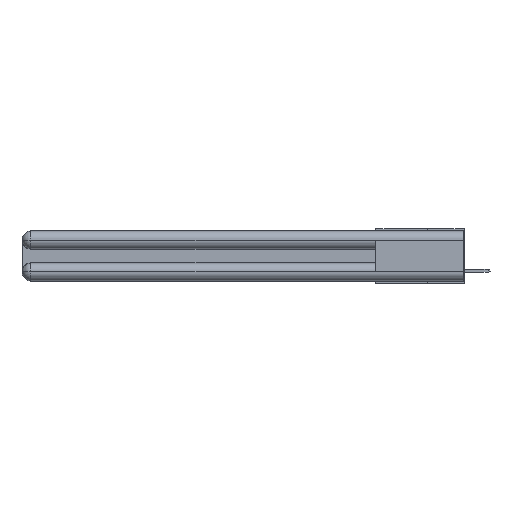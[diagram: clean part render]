
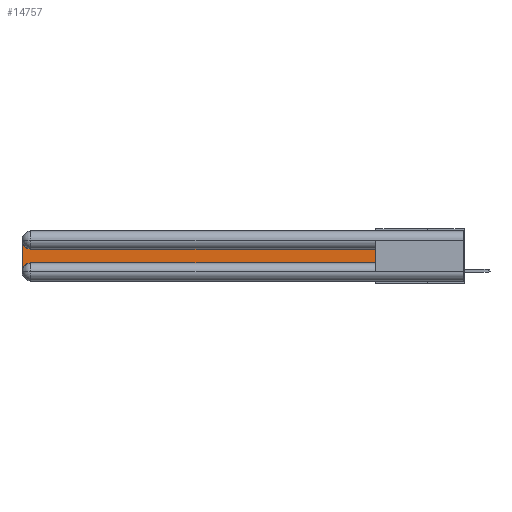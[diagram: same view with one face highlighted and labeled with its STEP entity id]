
A CAD part, left-side view. The second image highlights one B-rep face of the part: STEP entity #14757.
In plain terms, the highlighted planar face has unit normal (-1, 0, 0).
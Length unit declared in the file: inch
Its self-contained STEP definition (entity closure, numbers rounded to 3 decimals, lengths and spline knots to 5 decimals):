
#2024 = EDGE_LOOP ( 'NONE', ( #2301, #30990, #30283, #21975, #24722, #20316 ) ) ;
#2221 = CARTESIAN_POINT ( 'NONE',  ( 0.075, 3., -0.0625 ) ) ;
#2287 = AXIS2_PLACEMENT_3D ( 'NONE', #23627, #3652, #10839 ) ;
#2301 = ORIENTED_EDGE ( 'NONE', *, *, #5754, .T. ) ;
#2393 = VECTOR ( 'NONE', #24924, 39.37008 ) ;
#2893 = LINE ( 'NONE', #19226, #31942 ) ;
#3136 = DIRECTION ( 'NONE',  ( 0., 0., -1. ) ) ;
#3536 = EDGE_CURVE ( 'NONE', #25233, #27557, #24009, .T. ) ;
#3552 = DIRECTION ( 'NONE',  ( 0., 0., -1. ) ) ;
#3652 = DIRECTION ( 'NONE',  ( 1., 0., 0. ) ) ;
#4412 = EDGE_CURVE ( 'NONE', #13787, #19863, #2893, .T. ) ;
#5197 = EDGE_CURVE ( 'NONE', #27557, #18472, #24568, .T. ) ;
#5565 = AXIS2_PLACEMENT_3D ( 'NONE', #30758, #15905, #3552 ) ;
#5754 = EDGE_CURVE ( 'NONE', #18472, #8360, #21845, .T. ) ;
#6960 = EDGE_CURVE ( 'NONE', #8360, #13787, #17496, .T. ) ;
#7767 = CARTESIAN_POINT ( 'NONE',  ( 0.075, 0.6, -0.2175 ) ) ;
#8360 = VERTEX_POINT ( 'NONE', #31097 ) ;
#10649 = DIRECTION ( 'NONE',  ( 0., 0., 1. ) ) ;
#10839 = DIRECTION ( 'NONE',  ( 0., 0., -1. ) ) ;
#13787 = VERTEX_POINT ( 'NONE', #2221 ) ;
#13825 = AXIS2_PLACEMENT_3D ( 'NONE', #22681, #27758, #3136 ) ;
#14757 = ADVANCED_FACE ( 'NONE', ( #28942 ), #28274, .F. ) ;
#15905 = DIRECTION ( 'NONE',  ( 1., 0., 0. ) ) ;
#16246 = CIRCLE ( 'NONE', #5565, 0.06 ) ;
#17496 = CIRCLE ( 'NONE', #13825, 0.06 ) ;
#18472 = VERTEX_POINT ( 'NONE', #29125 ) ;
#19007 = DIRECTION ( 'NONE',  ( 0., 0., -1. ) ) ;
#19226 = CARTESIAN_POINT ( 'NONE',  ( 0.075, 3., -0.2175 ) ) ;
#19616 = CARTESIAN_POINT ( 'NONE',  ( 0.075, 2.94, -0.2175 ) ) ;
#19863 = VERTEX_POINT ( 'NONE', #24885 ) ;
#20316 = ORIENTED_EDGE ( 'NONE', *, *, #5197, .T. ) ;
#21845 = LINE ( 'NONE', #30002, #2393 ) ;
#21975 = ORIENTED_EDGE ( 'NONE', *, *, #22441, .T. ) ;
#22441 = EDGE_CURVE ( 'NONE', #19863, #25233, #16246, .T. ) ;
#22681 = CARTESIAN_POINT ( 'NONE',  ( 0.075, 2.94, -0.0625 ) ) ;
#23601 = VECTOR ( 'NONE', #24399, 39.37008 ) ;
#23627 = CARTESIAN_POINT ( 'NONE',  ( 0.075, 3., -0.1225 ) ) ;
#24009 = LINE ( 'NONE', #24292, #23601 ) ;
#24292 = CARTESIAN_POINT ( 'NONE',  ( 0.075, 0.6, -0.2175 ) ) ;
#24399 = DIRECTION ( 'NONE',  ( 0., -1., 0. ) ) ;
#24568 = LINE ( 'NONE', #27558, #28828 ) ;
#24722 = ORIENTED_EDGE ( 'NONE', *, *, #3536, .T. ) ;
#24885 = CARTESIAN_POINT ( 'NONE',  ( 0.075, 3., -0.2775 ) ) ;
#24924 = DIRECTION ( 'NONE',  ( 0., 1., 0. ) ) ;
#25233 = VERTEX_POINT ( 'NONE', #19616 ) ;
#27557 = VERTEX_POINT ( 'NONE', #7767 ) ;
#27558 = CARTESIAN_POINT ( 'NONE',  ( 0.075, 0.6, -0.2175 ) ) ;
#27758 = DIRECTION ( 'NONE',  ( 1., 0., 0. ) ) ;
#28274 = PLANE ( 'NONE',  #2287 ) ;
#28828 = VECTOR ( 'NONE', #10649, 39.37008 ) ;
#28942 = FACE_OUTER_BOUND ( 'NONE', #2024, .T. ) ;
#29125 = CARTESIAN_POINT ( 'NONE',  ( 0.075, 0.6, -0.1225 ) ) ;
#30002 = CARTESIAN_POINT ( 'NONE',  ( 0.075, 0.6, -0.1225 ) ) ;
#30283 = ORIENTED_EDGE ( 'NONE', *, *, #4412, .T. ) ;
#30758 = CARTESIAN_POINT ( 'NONE',  ( 0.075, 2.94, -0.2775 ) ) ;
#30990 = ORIENTED_EDGE ( 'NONE', *, *, #6960, .T. ) ;
#31097 = CARTESIAN_POINT ( 'NONE',  ( 0.075, 2.94, -0.1225 ) ) ;
#31942 = VECTOR ( 'NONE', #19007, 39.37008 ) ;
